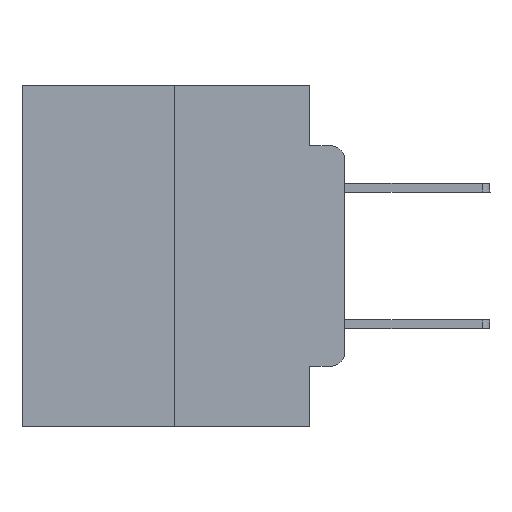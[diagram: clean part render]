
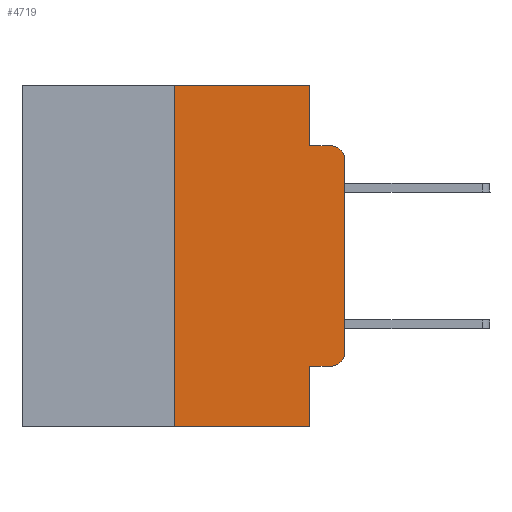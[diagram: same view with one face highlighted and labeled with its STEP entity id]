
A CAD part, left-side view. The second image highlights one B-rep face of the part: STEP entity #4719.
In plain terms, the highlighted planar face has unit normal (-1, 0, 0).
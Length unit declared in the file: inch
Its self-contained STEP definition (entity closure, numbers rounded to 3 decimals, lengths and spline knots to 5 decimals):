
#146 = CARTESIAN_POINT ( 'NONE',  ( 0., 0.02, -0.1085 ) ) ;
#276 = ORIENTED_EDGE ( 'NONE', *, *, #25958, .T. ) ;
#771 = ORIENTED_EDGE ( 'NONE', *, *, #5558, .F. ) ;
#826 = ORIENTED_EDGE ( 'NONE', *, *, #22067, .T. ) ;
#1440 = CIRCLE ( 'NONE', #18327, 0.02 ) ;
#3131 = EDGE_CURVE ( 'NONE', #9099, #24412, #22744, .T. ) ;
#3383 = CARTESIAN_POINT ( 'NONE',  ( 0., 0.051, 0. ) ) ;
#3858 = ORIENTED_EDGE ( 'NONE', *, *, #24767, .T. ) ;
#4331 = VECTOR ( 'NONE', #18587, 39.37008 ) ;
#4719 = ADVANCED_FACE ( 'NONE', ( #24147 ), #12009, .F. ) ;
#4812 = VECTOR ( 'NONE', #22951, 39.37008 ) ;
#4973 = VECTOR ( 'NONE', #9398, 39.37008 ) ;
#5071 = CIRCLE ( 'NONE', #21065, 0.02 ) ;
#5188 = CARTESIAN_POINT ( 'NONE',  ( 0., 0.473, -0.5 ) ) ;
#5464 = VERTEX_POINT ( 'NONE', #10056 ) ;
#5558 = EDGE_CURVE ( 'NONE', #22721, #9099, #8147, .T. ) ;
#5560 = LINE ( 'NONE', #20940, #17979 ) ;
#5872 = CARTESIAN_POINT ( 'NONE',  ( 0., 0.051, 0. ) ) ;
#5887 = CARTESIAN_POINT ( 'NONE',  ( 0., 0.473, 0. ) ) ;
#6185 = CARTESIAN_POINT ( 'NONE',  ( 0., 0.473, 0. ) ) ;
#6690 = CARTESIAN_POINT ( 'NONE',  ( 0., 0.02, -0.3915 ) ) ;
#6913 = LINE ( 'NONE', #25030, #23887 ) ;
#7705 = VERTEX_POINT ( 'NONE', #11578 ) ;
#8147 = LINE ( 'NONE', #24088, #26723 ) ;
#8169 = CARTESIAN_POINT ( 'NONE',  ( 0., 0., -0.3915 ) ) ;
#8211 = LINE ( 'NONE', #13096, #15377 ) ;
#9099 = VERTEX_POINT ( 'NONE', #21504 ) ;
#9398 = DIRECTION ( 'NONE',  ( 0., -1., 0. ) ) ;
#9949 = ORIENTED_EDGE ( 'NONE', *, *, #22161, .F. ) ;
#10056 = CARTESIAN_POINT ( 'NONE',  ( 0., 0.02, -0.0885 ) ) ;
#10071 = EDGE_CURVE ( 'NONE', #22391, #5464, #10661, .T. ) ;
#10375 = DIRECTION ( 'NONE',  ( 0., 0., 1. ) ) ;
#10661 = LINE ( 'NONE', #23545, #26619 ) ;
#10992 = ORIENTED_EDGE ( 'NONE', *, *, #20632, .F. ) ;
#11578 = CARTESIAN_POINT ( 'NONE',  ( 0., 0., -0.1085 ) ) ;
#12009 = PLANE ( 'NONE',  #17318 ) ;
#12718 = EDGE_LOOP ( 'NONE', ( #826, #26963, #20252, #9949, #18289, #771, #276, #10992, #23636, #3858 ) ) ;
#12728 = CARTESIAN_POINT ( 'NONE',  ( 0., 0.051, -0.4115 ) ) ;
#12974 = VERTEX_POINT ( 'NONE', #8169 ) ;
#12984 = DIRECTION ( 'NONE',  ( -1., 0., 0. ) ) ;
#12991 = CARTESIAN_POINT ( 'NONE',  ( 0., 0.25, -0.5 ) ) ;
#13096 = CARTESIAN_POINT ( 'NONE',  ( 0., 0.051, 0. ) ) ;
#13758 = VERTEX_POINT ( 'NONE', #12728 ) ;
#14455 = DIRECTION ( 'NONE',  ( 0., -1., 0. ) ) ;
#15094 = DIRECTION ( 'NONE',  ( 0., 0., -1. ) ) ;
#15377 = VECTOR ( 'NONE', #17388, 39.37008 ) ;
#16761 = LINE ( 'NONE', #3383, #4331 ) ;
#17193 = CARTESIAN_POINT ( 'NONE',  ( 0., 0.02, -0.4115 ) ) ;
#17318 = AXIS2_PLACEMENT_3D ( 'NONE', #5887, #20472, #26766 ) ;
#17388 = DIRECTION ( 'NONE',  ( 0., 0., -1. ) ) ;
#17485 = VERTEX_POINT ( 'NONE', #19494 ) ;
#17979 = VECTOR ( 'NONE', #10375, 39.37008 ) ;
#18289 = ORIENTED_EDGE ( 'NONE', *, *, #3131, .F. ) ;
#18327 = AXIS2_PLACEMENT_3D ( 'NONE', #6690, #12984, #15094 ) ;
#18587 = DIRECTION ( 'NONE',  ( 0., 0., -1. ) ) ;
#19494 = CARTESIAN_POINT ( 'NONE',  ( 0., 0.051, -0.5 ) ) ;
#19805 = DIRECTION ( 'NONE',  ( 0., 0., 1. ) ) ;
#20252 = ORIENTED_EDGE ( 'NONE', *, *, #10071, .F. ) ;
#20472 = DIRECTION ( 'NONE',  ( 1., 0., 0. ) ) ;
#20632 = EDGE_CURVE ( 'NONE', #13758, #17485, #16761, .T. ) ;
#20662 = DIRECTION ( 'NONE',  ( 0., 0., -1. ) ) ;
#20940 = CARTESIAN_POINT ( 'NONE',  ( 0., 0., 0. ) ) ;
#21065 = AXIS2_PLACEMENT_3D ( 'NONE', #146, #25061, #20662 ) ;
#21392 = EDGE_CURVE ( 'NONE', #13758, #25086, #6913, .T. ) ;
#21426 = DIRECTION ( 'NONE',  ( 0., -1., 0. ) ) ;
#21504 = CARTESIAN_POINT ( 'NONE',  ( 0., 0.25, 0. ) ) ;
#22067 = EDGE_CURVE ( 'NONE', #12974, #7705, #5560, .T. ) ;
#22161 = EDGE_CURVE ( 'NONE', #24412, #22391, #8211, .T. ) ;
#22391 = VERTEX_POINT ( 'NONE', #25852 ) ;
#22578 = LINE ( 'NONE', #5188, #4973 ) ;
#22721 = VERTEX_POINT ( 'NONE', #12991 ) ;
#22744 = LINE ( 'NONE', #6185, #4812 ) ;
#22951 = DIRECTION ( 'NONE',  ( 0., -1., 0. ) ) ;
#23545 = CARTESIAN_POINT ( 'NONE',  ( 0., 0.051, -0.0885 ) ) ;
#23636 = ORIENTED_EDGE ( 'NONE', *, *, #21392, .T. ) ;
#23854 = EDGE_CURVE ( 'NONE', #7705, #5464, #5071, .T. ) ;
#23887 = VECTOR ( 'NONE', #14455, 39.37008 ) ;
#24088 = CARTESIAN_POINT ( 'NONE',  ( 0., 0.25, 0. ) ) ;
#24147 = FACE_OUTER_BOUND ( 'NONE', #12718, .T. ) ;
#24412 = VERTEX_POINT ( 'NONE', #5872 ) ;
#24767 = EDGE_CURVE ( 'NONE', #25086, #12974, #1440, .T. ) ;
#25030 = CARTESIAN_POINT ( 'NONE',  ( 0., 0.051, -0.4115 ) ) ;
#25061 = DIRECTION ( 'NONE',  ( -1., 0., 0. ) ) ;
#25086 = VERTEX_POINT ( 'NONE', #17193 ) ;
#25852 = CARTESIAN_POINT ( 'NONE',  ( 0., 0.051, -0.0885 ) ) ;
#25958 = EDGE_CURVE ( 'NONE', #22721, #17485, #22578, .T. ) ;
#26619 = VECTOR ( 'NONE', #21426, 39.37008 ) ;
#26723 = VECTOR ( 'NONE', #19805, 39.37008 ) ;
#26766 = DIRECTION ( 'NONE',  ( 0., 0., -1. ) ) ;
#26963 = ORIENTED_EDGE ( 'NONE', *, *, #23854, .T. ) ;
